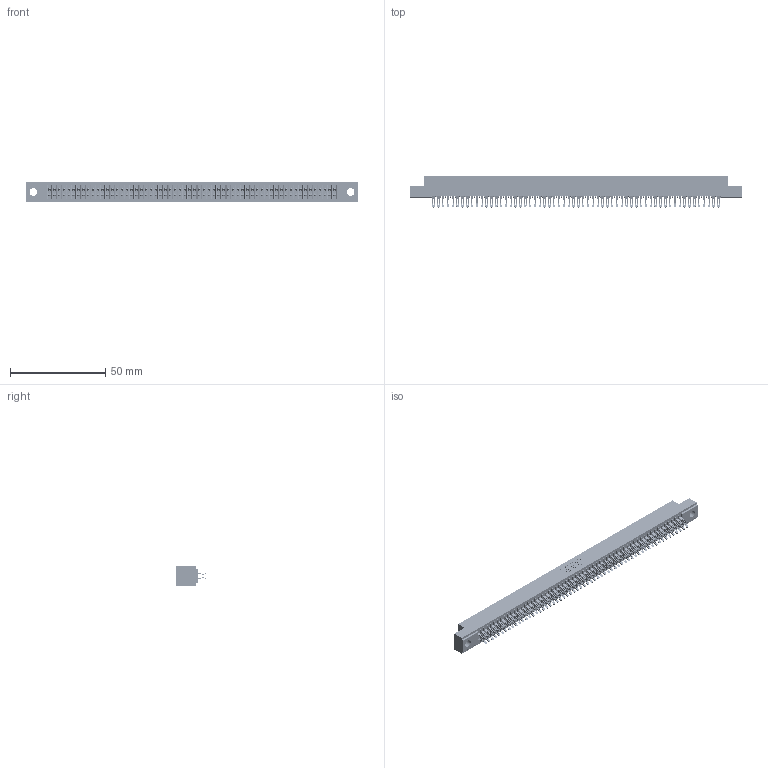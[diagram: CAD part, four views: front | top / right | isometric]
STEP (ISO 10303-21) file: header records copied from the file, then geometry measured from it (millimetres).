
FILE_DESCRIPTION (( 'STEP AP203' ), '1' );
FILE_NAME ('391-120-555-204.STEP', '2018-08-10T00:21:31', ( '' ), ( '' ), 'SwSTEP 2.0', 'SolidWorks 2016', '' );
FILE_SCHEMA (( 'CONFIG_CONTROL_DESIGN' ));
Products named in the file (3): 341 Part_.156 (3.96) Dia Mounting Holes; 341-292-001_341-292-155; 391-120-555-204
Assembly tree (121 placements, depth 2):
  391-120-555-204
    341 Part_.156 (3.96) Dia Mounting Holes
    341-292-001_341-292-155  x120
Bounding box: 174.62 x 16.31 x 10.16 mm (x, y, z)
Volume: 12957.6 mm3; surface area: 24435.4 mm2
Topology: 121 solids, 121 shells, 9490 faces, 28372 edges, 18470 vertices
Faces by surface type: plane 5122, cylinder 4128, sphere 122, torus 118
Entity records: 71103 total; most frequent: CARTESIAN_POINT 11840, ORIENTED_EDGE 11756, DIRECTION 11460, EDGE_CURVE 5878, LINE 4760, VECTOR 4760, VERTEX_POINT 3714, AXIS2_PLACEMENT_3D 3350
